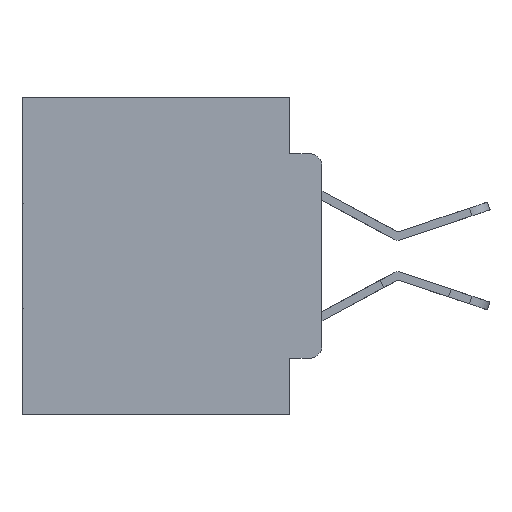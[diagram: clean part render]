
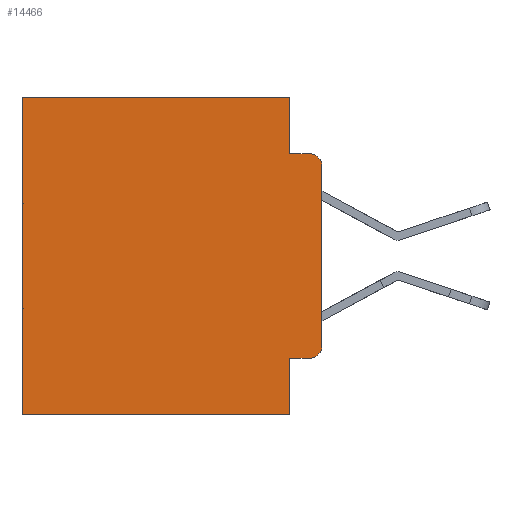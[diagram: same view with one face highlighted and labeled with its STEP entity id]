
A CAD part, left-side view. The second image highlights one B-rep face of the part: STEP entity #14466.
In plain terms, the highlighted planar face has unit normal (-1, 0, 0).
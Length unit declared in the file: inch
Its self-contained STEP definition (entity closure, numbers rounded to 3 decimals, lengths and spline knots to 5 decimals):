
#537 = VECTOR ( 'NONE', #11118, 39.37008 ) ;
#742 = DIRECTION ( 'NONE',  ( 0., 1., 0. ) ) ;
#1007 = CARTESIAN_POINT ( 'NONE',  ( 0.298, 0.02, -0.0885 ) ) ;
#1241 = DIRECTION ( 'NONE',  ( 0., 0., -1. ) ) ;
#1332 = LINE ( 'NONE', #6746, #19795 ) ;
#1403 = CARTESIAN_POINT ( 'NONE',  ( 0.298, 0.02, -0.1085 ) ) ;
#1651 = CARTESIAN_POINT ( 'NONE',  ( 0.298, 0.051, 0. ) ) ;
#1877 = VERTEX_POINT ( 'NONE', #1007 ) ;
#2342 = CIRCLE ( 'NONE', #5670, 0.02 ) ;
#2569 = ORIENTED_EDGE ( 'NONE', *, *, #29369, .T. ) ;
#2618 = VECTOR ( 'NONE', #26802, 39.37008 ) ;
#3079 = CARTESIAN_POINT ( 'NONE',  ( 0.298, 0.051, -0.0885 ) ) ;
#3905 = DIRECTION ( 'NONE',  ( 0., 0., -1. ) ) ;
#4143 = ORIENTED_EDGE ( 'NONE', *, *, #13810, .F. ) ;
#4150 = DIRECTION ( 'NONE',  ( 0., 0., -1. ) ) ;
#5330 = VECTOR ( 'NONE', #1241, 39.37008 ) ;
#5378 = VERTEX_POINT ( 'NONE', #25492 ) ;
#5553 = VERTEX_POINT ( 'NONE', #23073 ) ;
#5612 = DIRECTION ( 'NONE',  ( 0., -1., 0. ) ) ;
#5670 = AXIS2_PLACEMENT_3D ( 'NONE', #1403, #18321, #3905 ) ;
#5718 = EDGE_CURVE ( 'NONE', #14407, #5378, #21729, .T. ) ;
#6103 = LINE ( 'NONE', #24993, #5330 ) ;
#6240 = AXIS2_PLACEMENT_3D ( 'NONE', #10985, #27284, #13372 ) ;
#6746 = CARTESIAN_POINT ( 'NONE',  ( 0.298, 0.473, 0. ) ) ;
#7427 = EDGE_LOOP ( 'NONE', ( #29777, #2569, #28727, #25826, #28212, #10768, #24969, #4143, #7792, #25683 ) ) ;
#7653 = CARTESIAN_POINT ( 'NONE',  ( 0.298, 0.051, -0.5 ) ) ;
#7792 = ORIENTED_EDGE ( 'NONE', *, *, #5718, .T. ) ;
#7996 = PLANE ( 'NONE',  #13932 ) ;
#8206 = CARTESIAN_POINT ( 'NONE',  ( 0.298, 0., 0. ) ) ;
#8691 = CARTESIAN_POINT ( 'NONE',  ( 0.298, 0., 0. ) ) ;
#8885 = LINE ( 'NONE', #3079, #20685 ) ;
#10376 = VERTEX_POINT ( 'NONE', #14582 ) ;
#10768 = ORIENTED_EDGE ( 'NONE', *, *, #15390, .T. ) ;
#10979 = VERTEX_POINT ( 'NONE', #7653 ) ;
#10985 = CARTESIAN_POINT ( 'NONE',  ( 0.298, 0.02, -0.3915 ) ) ;
#11118 = DIRECTION ( 'NONE',  ( 0., 1., 0. ) ) ;
#11848 = VECTOR ( 'NONE', #742, 39.37008 ) ;
#12676 = CARTESIAN_POINT ( 'NONE',  ( 0.298, 0.473, -0.5 ) ) ;
#13038 = DIRECTION ( 'NONE',  ( 0., 0., -1. ) ) ;
#13223 = EDGE_CURVE ( 'NONE', #25692, #10376, #6103, .T. ) ;
#13372 = DIRECTION ( 'NONE',  ( 0., 0., -1. ) ) ;
#13546 = LINE ( 'NONE', #1651, #25170 ) ;
#13810 = EDGE_CURVE ( 'NONE', #14407, #10979, #15100, .T. ) ;
#13932 = AXIS2_PLACEMENT_3D ( 'NONE', #8206, #26951, #13038 ) ;
#14407 = VERTEX_POINT ( 'NONE', #22145 ) ;
#14466 = ADVANCED_FACE ( 'NONE', ( #27018 ), #7996, .F. ) ;
#14582 = CARTESIAN_POINT ( 'NONE',  ( 0.298, 0., -0.3915 ) ) ;
#15100 = LINE ( 'NONE', #26988, #21307 ) ;
#15390 = EDGE_CURVE ( 'NONE', #5553, #17923, #1332, .T. ) ;
#16647 = CARTESIAN_POINT ( 'NONE',  ( 0.298, 0.051, -0.0885 ) ) ;
#17923 = VERTEX_POINT ( 'NONE', #12676 ) ;
#18036 = CIRCLE ( 'NONE', #6240, 0.02 ) ;
#18321 = DIRECTION ( 'NONE',  ( -1., 0., 0. ) ) ;
#18377 = CARTESIAN_POINT ( 'NONE',  ( 0.298, 0., -0.1085 ) ) ;
#18911 = VERTEX_POINT ( 'NONE', #16647 ) ;
#19737 = VERTEX_POINT ( 'NONE', #29739 ) ;
#19755 = LINE ( 'NONE', #8691, #537 ) ;
#19795 = VECTOR ( 'NONE', #20955, 39.37008 ) ;
#20685 = VECTOR ( 'NONE', #5612, 39.37008 ) ;
#20955 = DIRECTION ( 'NONE',  ( 0., 0., -1. ) ) ;
#21307 = VECTOR ( 'NONE', #29316, 39.37008 ) ;
#21729 = LINE ( 'NONE', #26873, #2618 ) ;
#22145 = CARTESIAN_POINT ( 'NONE',  ( 0.298, 0.051, -0.4115 ) ) ;
#23073 = CARTESIAN_POINT ( 'NONE',  ( 0.298, 0.473, 0. ) ) ;
#23183 = EDGE_CURVE ( 'NONE', #19737, #18911, #13546, .T. ) ;
#23625 = EDGE_CURVE ( 'NONE', #19737, #5553, #19755, .T. ) ;
#24712 = EDGE_CURVE ( 'NONE', #18911, #1877, #8885, .T. ) ;
#24969 = ORIENTED_EDGE ( 'NONE', *, *, #25486, .F. ) ;
#24993 = CARTESIAN_POINT ( 'NONE',  ( 0.298, 0., 0. ) ) ;
#25170 = VECTOR ( 'NONE', #4150, 39.37008 ) ;
#25486 = EDGE_CURVE ( 'NONE', #10979, #17923, #30370, .T. ) ;
#25492 = CARTESIAN_POINT ( 'NONE',  ( 0.298, 0.02, -0.4115 ) ) ;
#25683 = ORIENTED_EDGE ( 'NONE', *, *, #26847, .T. ) ;
#25692 = VERTEX_POINT ( 'NONE', #18377 ) ;
#25826 = ORIENTED_EDGE ( 'NONE', *, *, #23183, .F. ) ;
#26802 = DIRECTION ( 'NONE',  ( 0., -1., 0. ) ) ;
#26847 = EDGE_CURVE ( 'NONE', #5378, #10376, #18036, .T. ) ;
#26873 = CARTESIAN_POINT ( 'NONE',  ( 0.298, 0.051, -0.4115 ) ) ;
#26951 = DIRECTION ( 'NONE',  ( 1., 0., 0. ) ) ;
#26988 = CARTESIAN_POINT ( 'NONE',  ( 0.298, 0.051, 0. ) ) ;
#27018 = FACE_OUTER_BOUND ( 'NONE', #7427, .T. ) ;
#27284 = DIRECTION ( 'NONE',  ( -1., 0., 0. ) ) ;
#28212 = ORIENTED_EDGE ( 'NONE', *, *, #23625, .T. ) ;
#28727 = ORIENTED_EDGE ( 'NONE', *, *, #24712, .F. ) ;
#29196 = CARTESIAN_POINT ( 'NONE',  ( 0.298, 0., -0.5 ) ) ;
#29316 = DIRECTION ( 'NONE',  ( 0., 0., -1. ) ) ;
#29369 = EDGE_CURVE ( 'NONE', #25692, #1877, #2342, .T. ) ;
#29739 = CARTESIAN_POINT ( 'NONE',  ( 0.298, 0.051, 0. ) ) ;
#29777 = ORIENTED_EDGE ( 'NONE', *, *, #13223, .F. ) ;
#30370 = LINE ( 'NONE', #29196, #11848 ) ;
